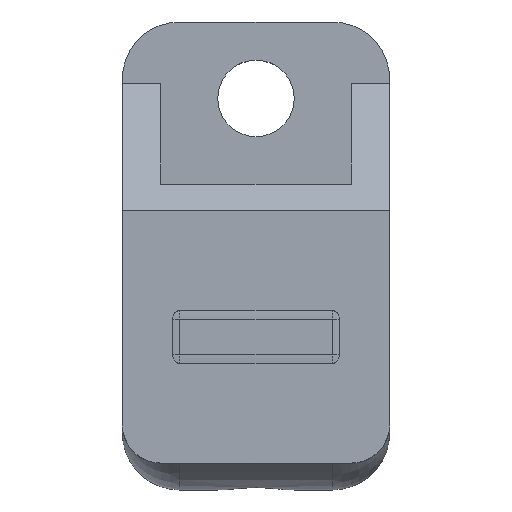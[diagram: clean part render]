
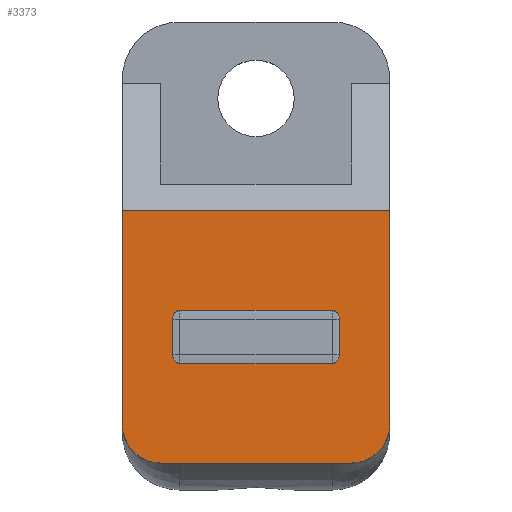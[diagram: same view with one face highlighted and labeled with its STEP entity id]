
A CAD part, top view. The second image highlights one B-rep face of the part: STEP entity #3373.
In plain terms, the highlighted planar face has unit normal (0, 0, 1).
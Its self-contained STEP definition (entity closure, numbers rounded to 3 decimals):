
#32 = VERTEX_POINT ( 'NONE', #1311 ) ;
#50 = CARTESIAN_POINT ( 'NONE',  ( -62.708, -12.6, 27.645 ) ) ;
#60 = VERTEX_POINT ( 'NONE', #3649 ) ;
#99 = CARTESIAN_POINT ( 'NONE',  ( -51.35, -20.13, 27.645 ) ) ;
#114 = ORIENTED_EDGE ( 'NONE', *, *, #536, .T. ) ;
#154 = DIRECTION ( 'NONE',  ( 0., -1., 0. ) ) ;
#245 = LINE ( 'NONE', #349, #1642 ) ;
#288 = ORIENTED_EDGE ( 'NONE', *, *, #2873, .F. ) ;
#295 = CARTESIAN_POINT ( 'NONE',  ( -63.35, -18.13, 27.645 ) ) ;
#303 = VERTEX_POINT ( 'NONE', #3464 ) ;
#307 = ORIENTED_EDGE ( 'NONE', *, *, #2530, .F. ) ;
#310 = CARTESIAN_POINT ( 'NONE',  ( -53.993, -12.6, 27.645 ) ) ;
#349 = CARTESIAN_POINT ( 'NONE',  ( -65.35, -20.13, 27.645 ) ) ;
#362 = DIRECTION ( 'NONE',  ( -1., 0., 0. ) ) ;
#363 = DIRECTION ( 'NONE',  ( 0., 1., 0. ) ) ;
#387 = VECTOR ( 'NONE', #403, 1000. ) ;
#392 = PLANE ( 'NONE',  #684 ) ;
#403 = DIRECTION ( 'NONE',  ( 0., 1., 0. ) ) ;
#481 = ORIENTED_EDGE ( 'NONE', *, *, #705, .F. ) ;
#485 = CARTESIAN_POINT ( 'NONE',  ( -53.35, -20.13, 27.645 ) ) ;
#492 = CARTESIAN_POINT ( 'NONE',  ( -58.35, -14.919, 27.645 ) ) ;
#518 = ORIENTED_EDGE ( 'NONE', *, *, #1933, .F. ) ;
#531 = EDGE_LOOP ( 'NONE', ( #1624, #518, #2665, #3346, #1082, #975, #2537, #481 ) ) ;
#536 = EDGE_CURVE ( 'NONE', #32, #1812, #2596, .T. ) ;
#617 = CARTESIAN_POINT ( 'NONE',  ( -62.56, -14.919, 27.645 ) ) ;
#619 = VERTEX_POINT ( 'NONE', #3698 ) ;
#661 = LINE ( 'NONE', #1510, #387 ) ;
#684 = AXIS2_PLACEMENT_3D ( 'NONE', #1545, #2062, #363 ) ;
#705 = EDGE_CURVE ( 'NONE', #303, #2199, #1274, .T. ) ;
#751 = FACE_BOUND ( 'NONE', #531, .T. ) ;
#844 = EDGE_CURVE ( 'NONE', #60, #1702, #1861, .T. ) ;
#897 = VERTEX_POINT ( 'NONE', #3593 ) ;
#911 = EDGE_CURVE ( 'NONE', #1463, #1099, #1631, .T. ) ;
#926 = CARTESIAN_POINT ( 'NONE',  ( -62.56, -12.138, 27.645 ) ) ;
#927 = ORIENTED_EDGE ( 'NONE', *, *, #2158, .T. ) ;
#929 = CIRCLE ( 'NONE', #1157, 2. ) ;
#975 = ORIENTED_EDGE ( 'NONE', *, *, #3315, .T. ) ;
#995 = VERTEX_POINT ( 'NONE', #3675 ) ;
#1064 = VECTOR ( 'NONE', #2678, 1000. ) ;
#1082 = ORIENTED_EDGE ( 'NONE', *, *, #2876, .T. ) ;
#1099 = VERTEX_POINT ( 'NONE', #485 ) ;
#1131 = EDGE_CURVE ( 'NONE', #2199, #995, #1434, .T. ) ;
#1153 = CARTESIAN_POINT ( 'NONE',  ( -54.35, -12.138, 27.645 ) ) ;
#1157 = AXIS2_PLACEMENT_3D ( 'NONE', #295, #1995, #1786 ) ;
#1167 = DIRECTION ( 'NONE',  ( 0., 1., 0. ) ) ;
#1190 = LINE ( 'NONE', #99, #2109 ) ;
#1191 = CARTESIAN_POINT ( 'NONE',  ( -54.141, -12.138, 27.645 ) ) ;
#1274 = LINE ( 'NONE', #3450, #2591 ) ;
#1293 = CARTESIAN_POINT ( 'NONE',  ( -51.35, -20.13, 27.645 ) ) ;
#1301 = DIRECTION ( 'NONE',  ( -1., 0., 0. ) ) ;
#1311 = CARTESIAN_POINT ( 'NONE',  ( -51.35, -6.91, 27.645 ) ) ;
#1325 = VECTOR ( 'NONE', #1301, 1000. ) ;
#1434 =( BOUNDED_CURVE ( )  B_SPLINE_CURVE ( 3, ( #3202, #926, #2836, #50 ),
 .UNSPECIFIED., .F., .T. ) 
 B_SPLINE_CURVE_WITH_KNOTS ( ( 4, 4 ),
 ( 3.138, 4.706 ),
 .UNSPECIFIED. ) 
 CURVE ( )  GEOMETRIC_REPRESENTATION_ITEM ( )  RATIONAL_B_SPLINE_CURVE ( ( 1., 0.805, 0.805, 1. ) ) 
 REPRESENTATION_ITEM ( '' )  );
#1458 = CARTESIAN_POINT ( 'NONE',  ( -62.35, -14.919, 27.645 ) ) ;
#1460 = ORIENTED_EDGE ( 'NONE', *, *, #911, .F. ) ;
#1463 = VERTEX_POINT ( 'NONE', #3553 ) ;
#1467 = VERTEX_POINT ( 'NONE', #1829 ) ;
#1510 = CARTESIAN_POINT ( 'NONE',  ( -62.708, -21.529, 27.645 ) ) ;
#1513 = LINE ( 'NONE', #1293, #1064 ) ;
#1545 = CARTESIAN_POINT ( 'NONE',  ( -51.35, -20.13, 27.645 ) ) ;
#1603 = VECTOR ( 'NONE', #2190, 1000. ) ;
#1624 = ORIENTED_EDGE ( 'NONE', *, *, #2898, .T. ) ;
#1631 = CIRCLE ( 'NONE', #2353, 2. ) ;
#1642 = VECTOR ( 'NONE', #1167, 1000. ) ;
#1702 = VERTEX_POINT ( 'NONE', #2316 ) ;
#1727 = DIRECTION ( 'NONE',  ( -1., 0., 0. ) ) ;
#1742 = CARTESIAN_POINT ( 'NONE',  ( -54.141, -14.919, 27.645 ) ) ;
#1743 = CARTESIAN_POINT ( 'NONE',  ( -62.708, -14.728, 27.645 ) ) ;
#1774 = CARTESIAN_POINT ( 'NONE',  ( -53.993, -14.458, 27.645 ) ) ;
#1786 = DIRECTION ( 'NONE',  ( 0., -1., 0. ) ) ;
#1812 = VERTEX_POINT ( 'NONE', #2753 ) ;
#1829 = CARTESIAN_POINT ( 'NONE',  ( -53.993, -12.6, 27.645 ) ) ;
#1841 = CARTESIAN_POINT ( 'NONE',  ( -51.35, -6.91, 27.645 ) ) ;
#1861 =( BOUNDED_CURVE ( )  B_SPLINE_CURVE ( 3, ( #2923, #1742, #2586, #1774 ),
 .UNSPECIFIED., .F., .T. ) 
 B_SPLINE_CURVE_WITH_KNOTS ( ( 4, 4 ),
 ( 6.279, 7.847 ),
 .UNSPECIFIED. ) 
 CURVE ( )  GEOMETRIC_REPRESENTATION_ITEM ( )  RATIONAL_B_SPLINE_CURVE ( ( 1., 0.805, 0.805, 1. ) ) 
 REPRESENTATION_ITEM ( '' )  );
#1933 = EDGE_CURVE ( 'NONE', #1702, #1467, #2400, .T. ) ;
#1988 = LINE ( 'NONE', #492, #1603 ) ;
#1995 = DIRECTION ( 'NONE',  ( 0., 0., -1. ) ) ;
#2062 = DIRECTION ( 'NONE',  ( 0., 0., -1. ) ) ;
#2109 = VECTOR ( 'NONE', #362, 1000. ) ;
#2158 = EDGE_CURVE ( 'NONE', #1463, #32, #1513, .T. ) ;
#2190 = DIRECTION ( 'NONE',  ( -1., 0., 0. ) ) ;
#2199 = VERTEX_POINT ( 'NONE', #2606 ) ;
#2253 = CARTESIAN_POINT ( 'NONE',  ( -62.35, -14.919, 27.645 ) ) ;
#2316 = CARTESIAN_POINT ( 'NONE',  ( -53.993, -14.458, 27.645 ) ) ;
#2331 = EDGE_CURVE ( 'NONE', #897, #2951, #929, .T. ) ;
#2353 = AXIS2_PLACEMENT_3D ( 'NONE', #3327, #2734, #154 ) ;
#2400 = LINE ( 'NONE', #2483, #3504 ) ;
#2483 = CARTESIAN_POINT ( 'NONE',  ( -53.993, -21.529, 27.645 ) ) ;
#2530 = EDGE_CURVE ( 'NONE', #1099, #897, #1190, .T. ) ;
#2537 = ORIENTED_EDGE ( 'NONE', *, *, #1131, .F. ) ;
#2579 =( BOUNDED_CURVE ( )  B_SPLINE_CURVE ( 3, ( #1153, #1191, #3163, #310 ),
 .UNSPECIFIED., .F., .F. ) 
 B_SPLINE_CURVE_WITH_KNOTS ( ( 4, 4 ),
 ( 6.279, 7.847 ),
 .UNSPECIFIED. ) 
 CURVE ( )  GEOMETRIC_REPRESENTATION_ITEM ( )  RATIONAL_B_SPLINE_CURVE ( ( 1., 0.805, 0.805, 1. ) ) 
 REPRESENTATION_ITEM ( '' )  );
#2586 = CARTESIAN_POINT ( 'NONE',  ( -53.993, -14.728, 27.645 ) ) ;
#2591 = VECTOR ( 'NONE', #1727, 1000. ) ;
#2596 = LINE ( 'NONE', #1841, #1325 ) ;
#2598 = CARTESIAN_POINT ( 'NONE',  ( -62.708, -14.458, 27.645 ) ) ;
#2606 = CARTESIAN_POINT ( 'NONE',  ( -62.35, -12.138, 27.645 ) ) ;
#2665 = ORIENTED_EDGE ( 'NONE', *, *, #844, .F. ) ;
#2678 = DIRECTION ( 'NONE',  ( 0., 1., 0. ) ) ;
#2734 = DIRECTION ( 'NONE',  ( 0., 0., -1. ) ) ;
#2753 = CARTESIAN_POINT ( 'NONE',  ( -65.35, -6.91, 27.645 ) ) ;
#2823 = DIRECTION ( 'NONE',  ( 0., 1., 0. ) ) ;
#2836 = CARTESIAN_POINT ( 'NONE',  ( -62.708, -12.329, 27.645 ) ) ;
#2873 = EDGE_CURVE ( 'NONE', #2951, #1812, #245, .T. ) ;
#2876 = EDGE_CURVE ( 'NONE', #3567, #619, #2913, .T. ) ;
#2898 = EDGE_CURVE ( 'NONE', #303, #1467, #2579, .T. ) ;
#2913 =( BOUNDED_CURVE ( )  B_SPLINE_CURVE ( 3, ( #1458, #617, #1743, #2598 ),
 .UNSPECIFIED., .F., .F. ) 
 B_SPLINE_CURVE_WITH_KNOTS ( ( 4, 4 ),
 ( 3.138, 4.706 ),
 .UNSPECIFIED. ) 
 CURVE ( )  GEOMETRIC_REPRESENTATION_ITEM ( )  RATIONAL_B_SPLINE_CURVE ( ( 1., 0.805, 0.805, 1. ) ) 
 REPRESENTATION_ITEM ( '' )  );
#2923 = CARTESIAN_POINT ( 'NONE',  ( -54.35, -14.919, 27.645 ) ) ;
#2951 = VERTEX_POINT ( 'NONE', #3496 ) ;
#3163 = CARTESIAN_POINT ( 'NONE',  ( -53.993, -12.329, 27.645 ) ) ;
#3202 = CARTESIAN_POINT ( 'NONE',  ( -62.35, -12.138, 27.645 ) ) ;
#3212 = FACE_OUTER_BOUND ( 'NONE', #3356, .T. ) ;
#3268 = ORIENTED_EDGE ( 'NONE', *, *, #2331, .F. ) ;
#3315 = EDGE_CURVE ( 'NONE', #619, #995, #661, .T. ) ;
#3327 = CARTESIAN_POINT ( 'NONE',  ( -53.35, -18.13, 27.645 ) ) ;
#3346 = ORIENTED_EDGE ( 'NONE', *, *, #3419, .T. ) ;
#3356 = EDGE_LOOP ( 'NONE', ( #307, #1460, #927, #114, #288, #3268 ) ) ;
#3373 = ADVANCED_FACE ( 'NONE', ( #3212, #751 ), #392, .F. ) ;
#3419 = EDGE_CURVE ( 'NONE', #60, #3567, #1988, .T. ) ;
#3450 = CARTESIAN_POINT ( 'NONE',  ( -58.35, -12.138, 27.645 ) ) ;
#3464 = CARTESIAN_POINT ( 'NONE',  ( -54.35, -12.138, 27.645 ) ) ;
#3496 = CARTESIAN_POINT ( 'NONE',  ( -65.35, -18.13, 27.645 ) ) ;
#3504 = VECTOR ( 'NONE', #2823, 1000. ) ;
#3553 = CARTESIAN_POINT ( 'NONE',  ( -51.35, -18.13, 27.645 ) ) ;
#3567 = VERTEX_POINT ( 'NONE', #2253 ) ;
#3593 = CARTESIAN_POINT ( 'NONE',  ( -63.35, -20.13, 27.645 ) ) ;
#3649 = CARTESIAN_POINT ( 'NONE',  ( -54.35, -14.919, 27.645 ) ) ;
#3675 = CARTESIAN_POINT ( 'NONE',  ( -62.708, -12.6, 27.645 ) ) ;
#3698 = CARTESIAN_POINT ( 'NONE',  ( -62.708, -14.458, 27.645 ) ) ;
